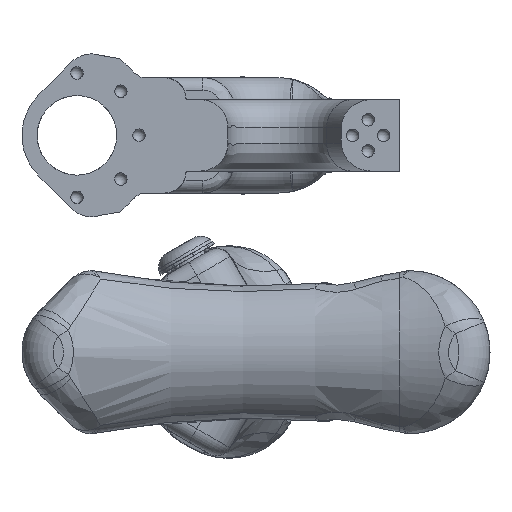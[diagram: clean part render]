
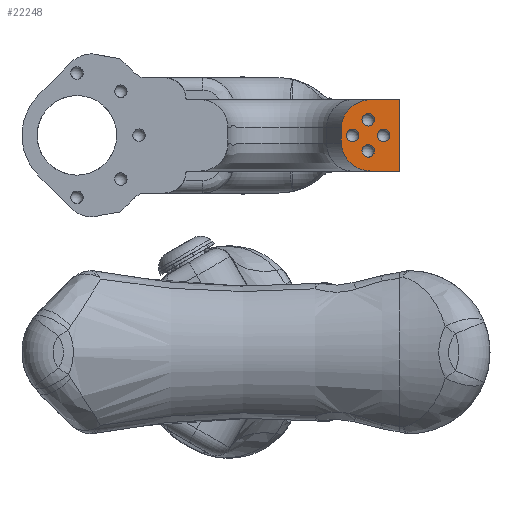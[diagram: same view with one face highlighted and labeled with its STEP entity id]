
A CAD part, front view. The second image highlights one B-rep face of the part: STEP entity #22248.
In plain terms, the highlighted planar face has unit normal (0, -1, 0).
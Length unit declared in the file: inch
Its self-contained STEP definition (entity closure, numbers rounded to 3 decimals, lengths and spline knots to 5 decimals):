
#1171 = ORIENTED_EDGE ( 'NONE', *, *, #58015, .F. ) ;
#2152 = CARTESIAN_POINT ( 'NONE',  ( -0.8556, -13.11147, 0.48539 ) ) ;
#3023 = CIRCLE ( 'NONE', #17770, 0.07874 ) ;
#4225 = EDGE_CURVE ( 'NONE', #19930, #77006, #6193, .T. ) ;
#5394 = EDGE_CURVE ( 'NONE', #66768, #21708, #73084, .T. ) ;
#6193 = LINE ( 'NONE', #68166, #20978 ) ;
#7306 = LINE ( 'NONE', #50662, #55558 ) ;
#7563 = CARTESIAN_POINT ( 'NONE',  ( -0.5166, -13.11147, -0.01782 ) ) ;
#11051 = ORIENTED_EDGE ( 'NONE', *, *, #5394, .T. ) ;
#11083 = ORIENTED_EDGE ( 'NONE', *, *, #24491, .F. ) ;
#11242 = DIRECTION ( 'NONE',  ( 0., 0., 1. ) ) ;
#11621 = CIRCLE ( 'NONE', #76926, 0.07874 ) ;
#11970 = VERTEX_POINT ( 'NONE', #73576 ) ;
#13196 = DIRECTION ( 'NONE',  ( -1., 0., 0. ) ) ;
#13277 = CIRCLE ( 'NONE', #41319, 0.07874 ) ;
#13867 = DIRECTION ( 'NONE',  ( 0., 0., 1. ) ) ;
#14151 = EDGE_LOOP ( 'NONE', ( #33580 ) ) ;
#16501 = CARTESIAN_POINT ( 'NONE',  ( -0.8556, -13.11147, 0.08024 ) ) ;
#17656 = VERTEX_POINT ( 'NONE', #40449 ) ;
#17770 = AXIS2_PLACEMENT_3D ( 'NONE', #23812, #67820, #30196 ) ;
#18747 = AXIS2_PLACEMENT_3D ( 'NONE', #29988, #48929, #11242 ) ;
#19670 = EDGE_CURVE ( 'NONE', #21708, #37925, #7306, .T. ) ;
#19831 = CARTESIAN_POINT ( 'NONE',  ( -0.5166, -13.11147, 0.06092 ) ) ;
#19930 = VERTEX_POINT ( 'NONE', #23602 ) ;
#20449 = CARTESIAN_POINT ( 'NONE',  ( -0.71345, -13.11147, 0.17903 ) ) ;
#20978 = VECTOR ( 'NONE', #74471, 39.37008 ) ;
#21150 = CARTESIAN_POINT ( 'NONE',  ( -0.47099, -13.11147, 0.63216 ) ) ;
#21708 = VERTEX_POINT ( 'NONE', #62009 ) ;
#21729 = CARTESIAN_POINT ( 'NONE',  ( -0.71345, -13.11147, 0.25777 ) ) ;
#22248 = ADVANCED_FACE ( 'NONE', ( #41694, #26931, #58427, #56439, #73152 ), #42617, .T. ) ;
#23079 = EDGE_CURVE ( 'NONE', #34529, #34529, #65183, .T. ) ;
#23602 = CARTESIAN_POINT ( 'NONE',  ( -0.47099, -13.11147, -0.27409 ) ) ;
#23812 = CARTESIAN_POINT ( 'NONE',  ( -0.5166, -13.11147, 0.37588 ) ) ;
#24054 = AXIS2_PLACEMENT_3D ( 'NONE', #7563, #51607, #13867 ) ;
#24491 = EDGE_CURVE ( 'NONE', #49255, #49255, #3023, .T. ) ;
#24877 = EDGE_LOOP ( 'NONE', ( #47025, #62070, #55837, #48582, #64873, #11051 ) ) ;
#25473 = DIRECTION ( 'NONE',  ( 0., 0., -1. ) ) ;
#25898 = CARTESIAN_POINT ( 'NONE',  ( 11.63933, -13.11147, 0.63216 ) ) ;
#26799 = DIRECTION ( 'NONE',  ( 0., 0., 1. ) ) ;
#26931 = FACE_BOUND ( 'NONE', #14151, .T. ) ;
#29207 = CARTESIAN_POINT ( 'NONE',  ( -0.69629, -13.11147, -0.27409 ) ) ;
#29988 = CARTESIAN_POINT ( 'NONE',  ( 11.63933, -13.11147, 44.02054 ) ) ;
#30196 = DIRECTION ( 'NONE',  ( 0., 0., 1. ) ) ;
#32550 = CARTESIAN_POINT ( 'NONE',  ( -0.5166, -13.11147, 0.45462 ) ) ;
#33323 = CARTESIAN_POINT ( 'NONE',  ( -0.31975, -13.11147, 0.17903 ) ) ;
#33580 = ORIENTED_EDGE ( 'NONE', *, *, #61406, .F. ) ;
#33586 = CARTESIAN_POINT ( 'NONE',  ( -0.69629, -13.11147, 0.63216 ) ) ;
#34529 = VERTEX_POINT ( 'NONE', #19831 ) ;
#37703 = EDGE_LOOP ( 'NONE', ( #11083 ) ) ;
#37925 = VERTEX_POINT ( 'NONE', #50672 ) ;
#39631 = DIRECTION ( 'NONE',  ( 0., 0., 1. ) ) ;
#40449 = CARTESIAN_POINT ( 'NONE',  ( -0.31975, -13.11147, 0.25777 ) ) ;
#41319 = AXIS2_PLACEMENT_3D ( 'NONE', #20449, #64455, #26799 ) ;
#41694 = FACE_BOUND ( 'NONE', #37703, .T. ) ;
#42617 = PLANE ( 'NONE',  #18747 ) ;
#45038 = EDGE_CURVE ( 'NONE', #11970, #66768, #77585, .T. ) ;
#47025 = ORIENTED_EDGE ( 'NONE', *, *, #19670, .T. ) ;
#48582 = ORIENTED_EDGE ( 'NONE', *, *, #67013, .F. ) ;
#48929 = DIRECTION ( 'NONE',  ( 0., -1., 0. ) ) ;
#49255 = VERTEX_POINT ( 'NONE', #32550 ) ;
#50109 = VECTOR ( 'NONE', #25473, 39.37008 ) ;
#50662 = CARTESIAN_POINT ( 'NONE',  ( -0.8556, -13.11147, 44.02054 ) ) ;
#50672 = CARTESIAN_POINT ( 'NONE',  ( -0.8556, -13.11147, 0.08024 ) ) ;
#51607 = DIRECTION ( 'NONE',  ( 0., -1., 0. ) ) ;
#52067 = LINE ( 'NONE', #63137, #50109 ) ;
#52217 = CARTESIAN_POINT ( 'NONE',  ( -0.47099, -13.11147, 0.63216 ) ) ;
#54220 = CARTESIAN_POINT ( 'NONE',  ( -0.8556, -13.11147, -0.12732 ) ) ;
#54654 = EDGE_CURVE ( 'NONE', #37925, #19930, #68841, .T. ) ;
#55558 = VECTOR ( 'NONE', #56968, 39.37008 ) ;
#55837 = ORIENTED_EDGE ( 'NONE', *, *, #4225, .T. ) ;
#56439 = FACE_BOUND ( 'NONE', #74648, .T. ) ;
#56968 = DIRECTION ( 'NONE',  ( 0., 0., -1. ) ) ;
#58015 = EDGE_CURVE ( 'NONE', #17656, #17656, #11621, .T. ) ;
#58427 = FACE_BOUND ( 'NONE', #73718, .T. ) ;
#58910 = VECTOR ( 'NONE', #13196, 39.37008 ) ;
#61406 = EDGE_CURVE ( 'NONE', #63919, #63919, #13277, .T. ) ;
#62009 = CARTESIAN_POINT ( 'NONE',  ( -0.8556, -13.11147, 0.27783 ) ) ;
#62070 = ORIENTED_EDGE ( 'NONE', *, *, #54654, .T. ) ;
#63137 = CARTESIAN_POINT ( 'NONE',  ( -0.1229, -13.11147, 18.04898 ) ) ;
#63919 = VERTEX_POINT ( 'NONE', #21729 ) ;
#64455 = DIRECTION ( 'NONE',  ( 0., -1., 0. ) ) ;
#64873 = ORIENTED_EDGE ( 'NONE', *, *, #45038, .T. ) ;
#65153 = CARTESIAN_POINT ( 'NONE',  ( -0.8556, -13.11147, 0.27783 ) ) ;
#65183 = CIRCLE ( 'NONE', #24054, 0.07874 ) ;
#66768 = VERTEX_POINT ( 'NONE', #52217 ) ;
#66892 = CARTESIAN_POINT ( 'NONE',  ( -0.1229, -13.11147, -0.27409 ) ) ;
#67013 = EDGE_CURVE ( 'NONE', #11970, #77006, #52067, .T. ) ;
#67820 = DIRECTION ( 'NONE',  ( 0., -1., 0. ) ) ;
#68166 = CARTESIAN_POINT ( 'NONE',  ( -3.32897, -13.11147, -0.27409 ) ) ;
#68841 =( BOUNDED_CURVE ( )  B_SPLINE_CURVE ( 3, ( #16501, #54220, #29207, #73159 ),
 .UNSPECIFIED., .F., .F. ) 
 B_SPLINE_CURVE_WITH_KNOTS ( ( 4, 4 ),
 ( 3.14159, 4.71239 ),
 .UNSPECIFIED. ) 
 CURVE ( )  GEOMETRIC_REPRESENTATION_ITEM ( )  RATIONAL_B_SPLINE_CURVE ( ( 1., 0.805, 0.805, 1. ) ) 
 REPRESENTATION_ITEM ( '' )  );
#72826 = ORIENTED_EDGE ( 'NONE', *, *, #23079, .F. ) ;
#73084 =( BOUNDED_CURVE ( )  B_SPLINE_CURVE ( 3, ( #21150, #33586, #2152, #65153 ),
 .UNSPECIFIED., .F., .F. ) 
 B_SPLINE_CURVE_WITH_KNOTS ( ( 4, 4 ),
 ( 4.71239, 6.28319 ),
 .UNSPECIFIED. ) 
 CURVE ( )  GEOMETRIC_REPRESENTATION_ITEM ( )  RATIONAL_B_SPLINE_CURVE ( ( 1., 0.805, 0.805, 1. ) ) 
 REPRESENTATION_ITEM ( '' )  );
#73152 = FACE_OUTER_BOUND ( 'NONE', #24877, .T. ) ;
#73159 = CARTESIAN_POINT ( 'NONE',  ( -0.47099, -13.11147, -0.27409 ) ) ;
#73576 = CARTESIAN_POINT ( 'NONE',  ( -0.1229, -13.11147, 0.63216 ) ) ;
#73718 = EDGE_LOOP ( 'NONE', ( #72826 ) ) ;
#74471 = DIRECTION ( 'NONE',  ( 1., 0., 0. ) ) ;
#74648 = EDGE_LOOP ( 'NONE', ( #1171 ) ) ;
#76926 = AXIS2_PLACEMENT_3D ( 'NONE', #33323, #77269, #39631 ) ;
#77006 = VERTEX_POINT ( 'NONE', #66892 ) ;
#77269 = DIRECTION ( 'NONE',  ( 0., -1., 0. ) ) ;
#77585 = LINE ( 'NONE', #25898, #58910 ) ;
